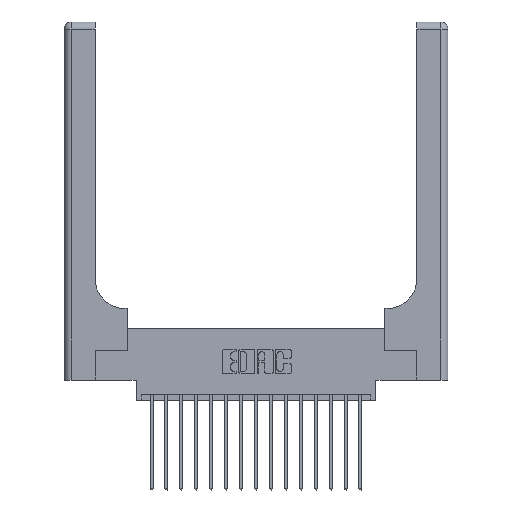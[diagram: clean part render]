
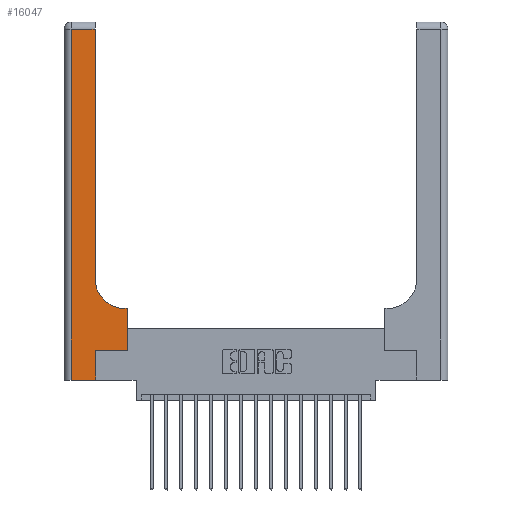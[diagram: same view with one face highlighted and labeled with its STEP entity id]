
A CAD part, top view. The second image highlights one B-rep face of the part: STEP entity #16047.
In plain terms, the highlighted planar face has unit normal (0, 0, 1).
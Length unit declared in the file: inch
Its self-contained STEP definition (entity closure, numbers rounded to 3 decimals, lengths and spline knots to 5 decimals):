
#30 = VECTOR ( 'NONE', #2229, 39.37008 ) ;
#539 = VECTOR ( 'NONE', #14056, 39.37008 ) ;
#683 = FACE_OUTER_BOUND ( 'NONE', #5061, .T. ) ;
#974 = VERTEX_POINT ( 'NONE', #2305 ) ;
#1278 = VECTOR ( 'NONE', #1950, 39.37008 ) ;
#1349 = VERTEX_POINT ( 'NONE', #15792 ) ;
#1558 = CARTESIAN_POINT ( 'NONE',  ( 0.265, 0., 0.37 ) ) ;
#1653 = CARTESIAN_POINT ( 'NONE',  ( 0.06, 2.94, 0.37 ) ) ;
#1689 = EDGE_CURVE ( 'NONE', #9028, #12306, #11671, .T. ) ;
#1714 = ORIENTED_EDGE ( 'NONE', *, *, #9445, .T. ) ;
#1950 = DIRECTION ( 'NONE',  ( -1., 0., 0. ) ) ;
#2229 = DIRECTION ( 'NONE',  ( 1., 0., 0. ) ) ;
#2293 = CARTESIAN_POINT ( 'NONE',  ( 0.265, 0.25, 0.37 ) ) ;
#2305 = CARTESIAN_POINT ( 'NONE',  ( 0.528, 0.25, 0.37 ) ) ;
#2365 = CARTESIAN_POINT ( 'NONE',  ( 0.26, 2.94, 0.37 ) ) ;
#3227 = ORIENTED_EDGE ( 'NONE', *, *, #1689, .T. ) ;
#3498 = LINE ( 'NONE', #4106, #10791 ) ;
#3914 = VERTEX_POINT ( 'NONE', #5261 ) ;
#4029 = EDGE_CURVE ( 'NONE', #974, #8942, #10897, .T. ) ;
#4085 = ORIENTED_EDGE ( 'NONE', *, *, #6905, .T. ) ;
#4106 = CARTESIAN_POINT ( 'NONE',  ( 0.06, 3., 0.37 ) ) ;
#4121 = ORIENTED_EDGE ( 'NONE', *, *, #9367, .T. ) ;
#4304 = DIRECTION ( 'NONE',  ( 0., 0., -1. ) ) ;
#4381 = CARTESIAN_POINT ( 'NONE',  ( 0.26, 0.85, 0.37 ) ) ;
#4410 = CARTESIAN_POINT ( 'NONE',  ( 0.265, 0., 0.37 ) ) ;
#4998 = VECTOR ( 'NONE', #6901, 39.37008 ) ;
#5059 = CARTESIAN_POINT ( 'NONE',  ( 0.06, 0., 0.37 ) ) ;
#5061 = EDGE_LOOP ( 'NONE', ( #3227, #4085, #1714, #7634, #14751, #7956, #6856, #4121, #15054 ) ) ;
#5261 = CARTESIAN_POINT ( 'NONE',  ( 0.265, 0.25, 0.37 ) ) ;
#5652 = CARTESIAN_POINT ( 'NONE',  ( 0.528, 0.6, 0.37 ) ) ;
#5654 = VERTEX_POINT ( 'NONE', #5059 ) ;
#5816 = CARTESIAN_POINT ( 'NONE',  ( 0.51, 0.85, 0.37 ) ) ;
#5989 = EDGE_CURVE ( 'NONE', #1349, #9028, #8156, .T. ) ;
#6039 = VERTEX_POINT ( 'NONE', #4410 ) ;
#6564 = VECTOR ( 'NONE', #9837, 39.37008 ) ;
#6856 = ORIENTED_EDGE ( 'NONE', *, *, #4029, .T. ) ;
#6901 = DIRECTION ( 'NONE',  ( 1., 0., 0. ) ) ;
#6905 = EDGE_CURVE ( 'NONE', #12306, #13766, #12878, .T. ) ;
#6919 = CARTESIAN_POINT ( 'NONE',  ( 0.528, 0.25, 0.37 ) ) ;
#7297 = DIRECTION ( 'NONE',  ( 1., 0., 0. ) ) ;
#7634 = ORIENTED_EDGE ( 'NONE', *, *, #16459, .T. ) ;
#7772 = AXIS2_PLACEMENT_3D ( 'NONE', #5816, #15974, #7297 ) ;
#7956 = ORIENTED_EDGE ( 'NONE', *, *, #15226, .T. ) ;
#7965 = LINE ( 'NONE', #15578, #4998 ) ;
#8050 = LINE ( 'NONE', #1558, #18665 ) ;
#8156 = CIRCLE ( 'NONE', #7772, 0.25 ) ;
#8246 = VECTOR ( 'NONE', #11450, 39.37008 ) ;
#8288 = LINE ( 'NONE', #12602, #539 ) ;
#8942 = VERTEX_POINT ( 'NONE', #5652 ) ;
#9028 = VERTEX_POINT ( 'NONE', #4381 ) ;
#9367 = EDGE_CURVE ( 'NONE', #8942, #1349, #8288, .T. ) ;
#9445 = EDGE_CURVE ( 'NONE', #13766, #5654, #3498, .T. ) ;
#9638 = EDGE_CURVE ( 'NONE', #6039, #3914, #8050, .T. ) ;
#9837 = DIRECTION ( 'NONE',  ( 0., 1., 0. ) ) ;
#10791 = VECTOR ( 'NONE', #12795, 39.37008 ) ;
#10897 = LINE ( 'NONE', #6919, #6564 ) ;
#11450 = DIRECTION ( 'NONE',  ( 0., 1., 0. ) ) ;
#11671 = LINE ( 'NONE', #12879, #8246 ) ;
#12086 = LINE ( 'NONE', #2293, #30 ) ;
#12306 = VERTEX_POINT ( 'NONE', #2365 ) ;
#12450 = AXIS2_PLACEMENT_3D ( 'NONE', #18600, #4304, #14439 ) ;
#12602 = CARTESIAN_POINT ( 'NONE',  ( 0.26, 0.6, 0.37 ) ) ;
#12795 = DIRECTION ( 'NONE',  ( 0., -1., 0. ) ) ;
#12878 = LINE ( 'NONE', #13704, #1278 ) ;
#12879 = CARTESIAN_POINT ( 'NONE',  ( 0.26, 3., 0.37 ) ) ;
#12997 = PLANE ( 'NONE',  #12450 ) ;
#13704 = CARTESIAN_POINT ( 'NONE',  ( 0., 2.94, 0.37 ) ) ;
#13766 = VERTEX_POINT ( 'NONE', #1653 ) ;
#14056 = DIRECTION ( 'NONE',  ( -1., 0., 0. ) ) ;
#14439 = DIRECTION ( 'NONE',  ( -1., 0., 0. ) ) ;
#14751 = ORIENTED_EDGE ( 'NONE', *, *, #9638, .T. ) ;
#15054 = ORIENTED_EDGE ( 'NONE', *, *, #5989, .T. ) ;
#15226 = EDGE_CURVE ( 'NONE', #3914, #974, #12086, .T. ) ;
#15578 = CARTESIAN_POINT ( 'NONE',  ( 0., 0., 0.37 ) ) ;
#15792 = CARTESIAN_POINT ( 'NONE',  ( 0.51, 0.6, 0.37 ) ) ;
#15974 = DIRECTION ( 'NONE',  ( 0., 0., -1. ) ) ;
#16047 = ADVANCED_FACE ( 'NONE', ( #683 ), #12997, .F. ) ;
#16112 = DIRECTION ( 'NONE',  ( 0., 1., 0. ) ) ;
#16459 = EDGE_CURVE ( 'NONE', #5654, #6039, #7965, .T. ) ;
#18600 = CARTESIAN_POINT ( 'NONE',  ( 0., 3., 0.37 ) ) ;
#18665 = VECTOR ( 'NONE', #16112, 39.37008 ) ;
